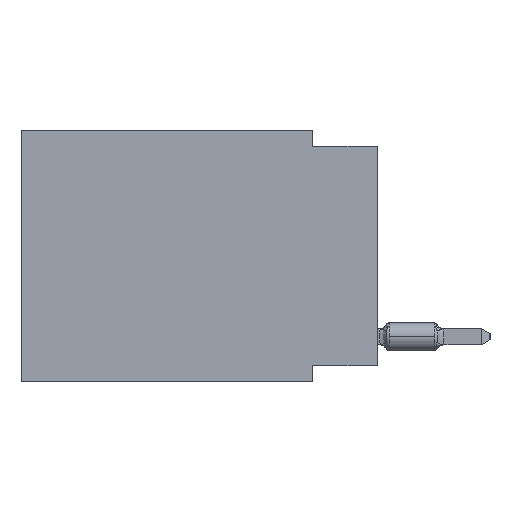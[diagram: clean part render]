
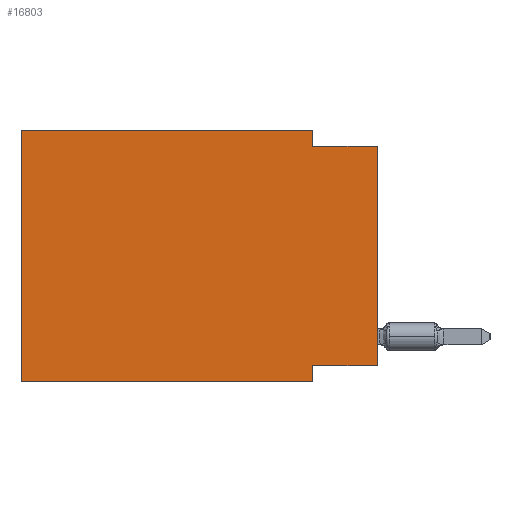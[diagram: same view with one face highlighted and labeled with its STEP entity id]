
A CAD part, left-side view. The second image highlights one B-rep face of the part: STEP entity #16803.
In plain terms, the highlighted planar face has unit normal (-1, 0, 0).
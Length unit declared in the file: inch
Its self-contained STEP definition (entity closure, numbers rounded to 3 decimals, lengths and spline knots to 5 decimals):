
#612 = VERTEX_POINT ( 'NONE', #8021 ) ;
#739 = CARTESIAN_POINT ( 'NONE',  ( 0., 0., -0.365 ) ) ;
#1633 = LINE ( 'NONE', #16512, #5992 ) ;
#1787 = VERTEX_POINT ( 'NONE', #15471 ) ;
#2237 = CARTESIAN_POINT ( 'NONE',  ( 0., 0.55, 0. ) ) ;
#2380 = VECTOR ( 'NONE', #10287, 39.37008 ) ;
#2430 = DIRECTION ( 'NONE',  ( 0., 0., 1. ) ) ;
#3001 = EDGE_CURVE ( 'NONE', #14562, #15612, #5760, .T. ) ;
#3803 = EDGE_CURVE ( 'NONE', #1787, #612, #13363, .T. ) ;
#3969 = DIRECTION ( 'NONE',  ( 0., 1., 0. ) ) ;
#4197 = ORIENTED_EDGE ( 'NONE', *, *, #3001, .F. ) ;
#4324 = VERTEX_POINT ( 'NONE', #23171 ) ;
#4337 = ORIENTED_EDGE ( 'NONE', *, *, #3803, .F. ) ;
#5164 = VERTEX_POINT ( 'NONE', #17437 ) ;
#5760 = LINE ( 'NONE', #20423, #20870 ) ;
#5785 = DIRECTION ( 'NONE',  ( 0., 0., 1. ) ) ;
#5992 = VECTOR ( 'NONE', #8955, 39.37008 ) ;
#6015 = ORIENTED_EDGE ( 'NONE', *, *, #23297, .F. ) ;
#6685 = LINE ( 'NONE', #12329, #2380 ) ;
#6774 = CARTESIAN_POINT ( 'NONE',  ( 0., 0., 0. ) ) ;
#7085 = EDGE_CURVE ( 'NONE', #14562, #5164, #23349, .T. ) ;
#7145 = CARTESIAN_POINT ( 'NONE',  ( 0., 0.1, -0.365 ) ) ;
#7263 = PLANE ( 'NONE',  #15413 ) ;
#7641 = ORIENTED_EDGE ( 'NONE', *, *, #7085, .T. ) ;
#8021 = CARTESIAN_POINT ( 'NONE',  ( 0., 0.55, 0. ) ) ;
#8955 = DIRECTION ( 'NONE',  ( 0., -1., 0. ) ) ;
#9171 = CARTESIAN_POINT ( 'NONE',  ( 0., 0.55, 0. ) ) ;
#9498 = EDGE_CURVE ( 'NONE', #17169, #5164, #1633, .T. ) ;
#10287 = DIRECTION ( 'NONE',  ( 0., -1., 0. ) ) ;
#10840 = VECTOR ( 'NONE', #18212, 39.37008 ) ;
#10985 = DIRECTION ( 'NONE',  ( 0., 0., -1. ) ) ;
#11131 = EDGE_LOOP ( 'NONE', ( #7641, #12475, #6015, #23318, #4337, #14222, #19348, #4197 ) ) ;
#11357 = VECTOR ( 'NONE', #14442, 39.37008 ) ;
#12081 = VECTOR ( 'NONE', #16209, 39.37008 ) ;
#12296 = VECTOR ( 'NONE', #2430, 39.37008 ) ;
#12329 = CARTESIAN_POINT ( 'NONE',  ( 0., 0.55, -0.39 ) ) ;
#12475 = ORIENTED_EDGE ( 'NONE', *, *, #9498, .F. ) ;
#13023 = FACE_OUTER_BOUND ( 'NONE', #11131, .T. ) ;
#13363 = LINE ( 'NONE', #20695, #12296 ) ;
#14222 = ORIENTED_EDGE ( 'NONE', *, *, #17328, .T. ) ;
#14442 = DIRECTION ( 'NONE',  ( 0., 0., -1. ) ) ;
#14562 = VERTEX_POINT ( 'NONE', #739 ) ;
#14960 = CARTESIAN_POINT ( 'NONE',  ( 0., 0.1, -0.39 ) ) ;
#15413 = AXIS2_PLACEMENT_3D ( 'NONE', #9171, #16750, #10985 ) ;
#15471 = CARTESIAN_POINT ( 'NONE',  ( 0., 0.55, -0.39 ) ) ;
#15612 = VERTEX_POINT ( 'NONE', #7145 ) ;
#16209 = DIRECTION ( 'NONE',  ( 0., -1., 0. ) ) ;
#16343 = VECTOR ( 'NONE', #5785, 39.37008 ) ;
#16512 = CARTESIAN_POINT ( 'NONE',  ( 0., 0., -0.025 ) ) ;
#16750 = DIRECTION ( 'NONE',  ( 1., 0., 0. ) ) ;
#16803 = ADVANCED_FACE ( 'NONE', ( #13023 ), #7263, .F. ) ;
#17169 = VERTEX_POINT ( 'NONE', #21612 ) ;
#17328 = EDGE_CURVE ( 'NONE', #1787, #4324, #6685, .T. ) ;
#17437 = CARTESIAN_POINT ( 'NONE',  ( 0., 0., -0.025 ) ) ;
#17569 = EDGE_CURVE ( 'NONE', #15612, #4324, #22049, .T. ) ;
#18212 = DIRECTION ( 'NONE',  ( 0., 0., -1. ) ) ;
#18737 = EDGE_CURVE ( 'NONE', #612, #19514, #21967, .T. ) ;
#19348 = ORIENTED_EDGE ( 'NONE', *, *, #17569, .F. ) ;
#19514 = VERTEX_POINT ( 'NONE', #20312 ) ;
#19857 = LINE ( 'NONE', #23567, #11357 ) ;
#20312 = CARTESIAN_POINT ( 'NONE',  ( 0., 0.1, 0. ) ) ;
#20423 = CARTESIAN_POINT ( 'NONE',  ( 0., 0., -0.365 ) ) ;
#20695 = CARTESIAN_POINT ( 'NONE',  ( 0., 0.55, 0. ) ) ;
#20870 = VECTOR ( 'NONE', #3969, 39.37008 ) ;
#21612 = CARTESIAN_POINT ( 'NONE',  ( 0., 0.1, -0.025 ) ) ;
#21967 = LINE ( 'NONE', #2237, #12081 ) ;
#22049 = LINE ( 'NONE', #14960, #10840 ) ;
#23171 = CARTESIAN_POINT ( 'NONE',  ( 0., 0.1, -0.39 ) ) ;
#23297 = EDGE_CURVE ( 'NONE', #19514, #17169, #19857, .T. ) ;
#23318 = ORIENTED_EDGE ( 'NONE', *, *, #18737, .F. ) ;
#23349 = LINE ( 'NONE', #6774, #16343 ) ;
#23567 = CARTESIAN_POINT ( 'NONE',  ( 0., 0.1, 0. ) ) ;
